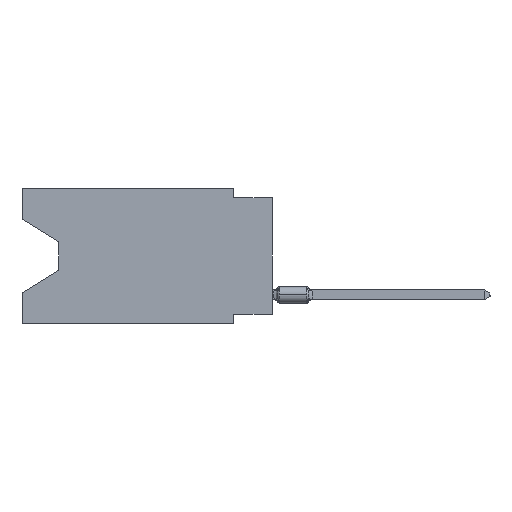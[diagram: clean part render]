
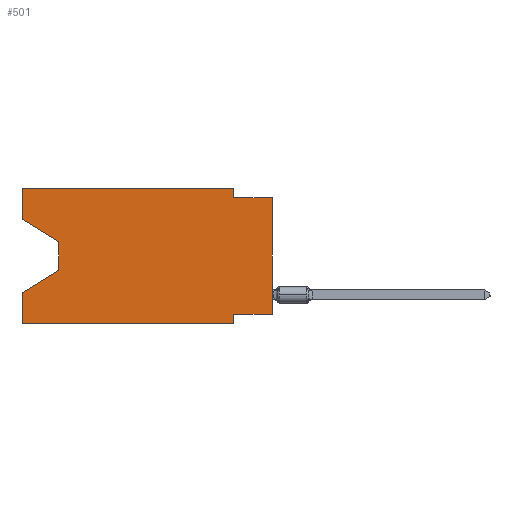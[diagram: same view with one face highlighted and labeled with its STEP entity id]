
A CAD part, left-side view. The second image highlights one B-rep face of the part: STEP entity #501.
In plain terms, the highlighted planar face has unit normal (-1, 0, 0).
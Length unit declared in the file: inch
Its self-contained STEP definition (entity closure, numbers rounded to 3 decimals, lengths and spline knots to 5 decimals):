
#85 = CARTESIAN_POINT ( 'NONE',  ( 0., 0.645, -0.35 ) ) ;
#299 = CARTESIAN_POINT ( 'NONE',  ( 0., 0., -0.325 ) ) ;
#501 = ADVANCED_FACE ( 'NONE', ( #7287 ), #16222, .F. ) ;
#518 = ORIENTED_EDGE ( 'NONE', *, *, #30371, .F. ) ;
#741 = VERTEX_POINT ( 'NONE', #29633 ) ;
#849 = LINE ( 'NONE', #17347, #2653 ) ;
#999 = ORIENTED_EDGE ( 'NONE', *, *, #26082, .T. ) ;
#1128 = EDGE_CURVE ( 'NONE', #29656, #13222, #3503, .T. ) ;
#1170 = DIRECTION ( 'NONE',  ( 0., -1., 0. ) ) ;
#1532 = CARTESIAN_POINT ( 'NONE',  ( 0., 0.55, -0.212 ) ) ;
#2257 = VERTEX_POINT ( 'NONE', #12227 ) ;
#2634 = VERTEX_POINT ( 'NONE', #299 ) ;
#2653 = VECTOR ( 'NONE', #29530, 39.37008 ) ;
#2675 = LINE ( 'NONE', #2989, #13001 ) ;
#2708 = DIRECTION ( 'NONE',  ( 0., 0., 1. ) ) ;
#2812 = VECTOR ( 'NONE', #7958, 39.37008 ) ;
#2919 = EDGE_CURVE ( 'NONE', #13464, #741, #25286, .T. ) ;
#2989 = CARTESIAN_POINT ( 'NONE',  ( 0., 0.55, -0.138 ) ) ;
#3503 = LINE ( 'NONE', #13032, #4899 ) ;
#3581 = DIRECTION ( 'NONE',  ( 0., -0.855, -0.519 ) ) ;
#3862 = DIRECTION ( 'NONE',  ( 0., 0.855, -0.519 ) ) ;
#3870 = ORIENTED_EDGE ( 'NONE', *, *, #22062, .F. ) ;
#4079 = CARTESIAN_POINT ( 'NONE',  ( 0., 0.1, -0.35 ) ) ;
#4396 = VERTEX_POINT ( 'NONE', #21959 ) ;
#4401 = EDGE_CURVE ( 'NONE', #2257, #741, #849, .T. ) ;
#4459 = DIRECTION ( 'NONE',  ( 0., 0., -1. ) ) ;
#4504 = EDGE_CURVE ( 'NONE', #18795, #20008, #27675, .T. ) ;
#4509 = CARTESIAN_POINT ( 'NONE',  ( 0., 0., -0.025 ) ) ;
#4899 = VECTOR ( 'NONE', #1170, 39.37008 ) ;
#5061 = LINE ( 'NONE', #23248, #16644 ) ;
#5598 = ORIENTED_EDGE ( 'NONE', *, *, #25709, .F. ) ;
#5610 = ORIENTED_EDGE ( 'NONE', *, *, #28703, .T. ) ;
#6331 = DIRECTION ( 'NONE',  ( 0., 0., 1. ) ) ;
#6573 = CARTESIAN_POINT ( 'NONE',  ( 0., 0.645, 0. ) ) ;
#6829 = DIRECTION ( 'NONE',  ( 0., 0., -1. ) ) ;
#7287 = FACE_OUTER_BOUND ( 'NONE', #9078, .T. ) ;
#7958 = DIRECTION ( 'NONE',  ( 0., 1., 0. ) ) ;
#8025 = ORIENTED_EDGE ( 'NONE', *, *, #14855, .T. ) ;
#9072 = ORIENTED_EDGE ( 'NONE', *, *, #4401, .F. ) ;
#9078 = EDGE_LOOP ( 'NONE', ( #8025, #999, #12657, #9072, #26188, #15405, #5598, #5610, #23118, #3870, #518, #25837 ) ) ;
#9444 = DIRECTION ( 'NONE',  ( 1., 0., 0. ) ) ;
#11974 = DIRECTION ( 'NONE',  ( 0., -1., 0. ) ) ;
#12227 = CARTESIAN_POINT ( 'NONE',  ( 0., 0.645, -0.35 ) ) ;
#12418 = LINE ( 'NONE', #26309, #25056 ) ;
#12657 = ORIENTED_EDGE ( 'NONE', *, *, #2919, .T. ) ;
#13001 = VECTOR ( 'NONE', #19007, 39.37008 ) ;
#13032 = CARTESIAN_POINT ( 'NONE',  ( 0., 0., -0.025 ) ) ;
#13107 = VECTOR ( 'NONE', #29418, 39.37008 ) ;
#13222 = VERTEX_POINT ( 'NONE', #4509 ) ;
#13464 = VERTEX_POINT ( 'NONE', #1532 ) ;
#13779 = VERTEX_POINT ( 'NONE', #23869 ) ;
#14424 = VECTOR ( 'NONE', #3581, 39.37008 ) ;
#14855 = EDGE_CURVE ( 'NONE', #13779, #21766, #23731, .T. ) ;
#15120 = AXIS2_PLACEMENT_3D ( 'NONE', #18378, #9444, #6829 ) ;
#15405 = ORIENTED_EDGE ( 'NONE', *, *, #4504, .F. ) ;
#15514 = CARTESIAN_POINT ( 'NONE',  ( 0., 0.55, -0.138 ) ) ;
#15607 = DIRECTION ( 'NONE',  ( 0., 0., -1. ) ) ;
#16222 = PLANE ( 'NONE',  #15120 ) ;
#16561 = EDGE_CURVE ( 'NONE', #2257, #20008, #29926, .T. ) ;
#16644 = VECTOR ( 'NONE', #4459, 39.37008 ) ;
#17347 = CARTESIAN_POINT ( 'NONE',  ( 0., 0.645, 0. ) ) ;
#17874 = VECTOR ( 'NONE', #11974, 39.37008 ) ;
#18378 = CARTESIAN_POINT ( 'NONE',  ( 0., 0.645, 0. ) ) ;
#18795 = VERTEX_POINT ( 'NONE', #28045 ) ;
#19007 = DIRECTION ( 'NONE',  ( 0., 0., -1. ) ) ;
#19674 = LINE ( 'NONE', #29092, #2812 ) ;
#20008 = VERTEX_POINT ( 'NONE', #27897 ) ;
#20530 = EDGE_CURVE ( 'NONE', #13779, #4396, #12418, .T. ) ;
#21766 = VERTEX_POINT ( 'NONE', #15514 ) ;
#21959 = CARTESIAN_POINT ( 'NONE',  ( 0., 0.645, 0. ) ) ;
#22062 = EDGE_CURVE ( 'NONE', #30090, #29656, #5061, .T. ) ;
#23118 = ORIENTED_EDGE ( 'NONE', *, *, #1128, .F. ) ;
#23248 = CARTESIAN_POINT ( 'NONE',  ( 0., 0.1, 0. ) ) ;
#23731 = LINE ( 'NONE', #27330, #14424 ) ;
#23869 = CARTESIAN_POINT ( 'NONE',  ( 0., 0.645, -0.08025 ) ) ;
#24005 = VECTOR ( 'NONE', #3862, 39.37008 ) ;
#24347 = VECTOR ( 'NONE', #15607, 39.37008 ) ;
#24542 = LINE ( 'NONE', #24992, #26359 ) ;
#24980 = CARTESIAN_POINT ( 'NONE',  ( 0., 0.55, -0.212 ) ) ;
#24992 = CARTESIAN_POINT ( 'NONE',  ( 0., 0., 0. ) ) ;
#25056 = VECTOR ( 'NONE', #2708, 39.37008 ) ;
#25286 = LINE ( 'NONE', #24980, #24005 ) ;
#25503 = CARTESIAN_POINT ( 'NONE',  ( 0., 0.1, -0.025 ) ) ;
#25709 = EDGE_CURVE ( 'NONE', #2634, #18795, #19674, .T. ) ;
#25837 = ORIENTED_EDGE ( 'NONE', *, *, #20530, .F. ) ;
#25915 = CARTESIAN_POINT ( 'NONE',  ( 0., 0.1, 0. ) ) ;
#26082 = EDGE_CURVE ( 'NONE', #21766, #13464, #2675, .T. ) ;
#26188 = ORIENTED_EDGE ( 'NONE', *, *, #16561, .T. ) ;
#26309 = CARTESIAN_POINT ( 'NONE',  ( 0., 0.645, 0. ) ) ;
#26359 = VECTOR ( 'NONE', #6331, 39.37008 ) ;
#27330 = CARTESIAN_POINT ( 'NONE',  ( 0., 0.645, -0.08025 ) ) ;
#27675 = LINE ( 'NONE', #4079, #24347 ) ;
#27897 = CARTESIAN_POINT ( 'NONE',  ( 0., 0.1, -0.35 ) ) ;
#28045 = CARTESIAN_POINT ( 'NONE',  ( 0., 0.1, -0.325 ) ) ;
#28703 = EDGE_CURVE ( 'NONE', #2634, #13222, #24542, .T. ) ;
#29092 = CARTESIAN_POINT ( 'NONE',  ( 0., 0., -0.325 ) ) ;
#29418 = DIRECTION ( 'NONE',  ( 0., -1., 0. ) ) ;
#29530 = DIRECTION ( 'NONE',  ( 0., 0., 1. ) ) ;
#29633 = CARTESIAN_POINT ( 'NONE',  ( 0., 0.645, -0.26975 ) ) ;
#29656 = VERTEX_POINT ( 'NONE', #25503 ) ;
#29926 = LINE ( 'NONE', #85, #17874 ) ;
#30035 = LINE ( 'NONE', #6573, #13107 ) ;
#30090 = VERTEX_POINT ( 'NONE', #25915 ) ;
#30371 = EDGE_CURVE ( 'NONE', #4396, #30090, #30035, .T. ) ;
